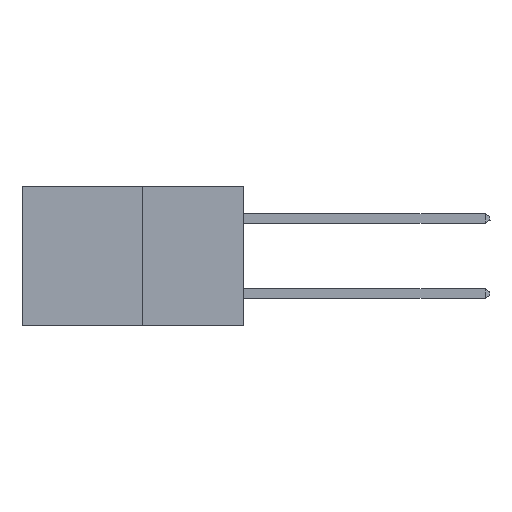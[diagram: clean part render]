
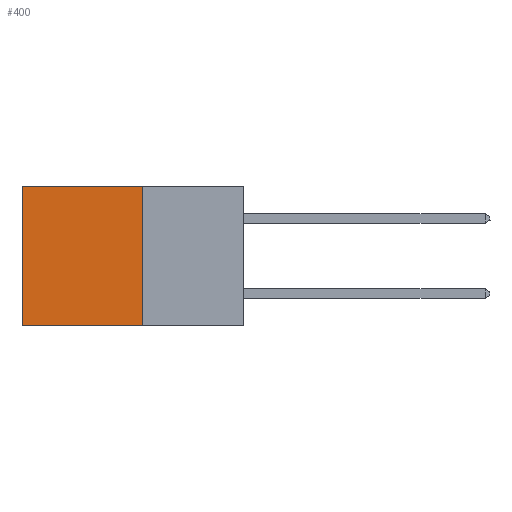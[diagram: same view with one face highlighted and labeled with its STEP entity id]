
A CAD part, left-side view. The second image highlights one B-rep face of the part: STEP entity #400.
In plain terms, the highlighted planar face has unit normal (-1, 0, 0).
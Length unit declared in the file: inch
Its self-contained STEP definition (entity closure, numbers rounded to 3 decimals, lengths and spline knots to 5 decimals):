
#313 = ORIENTED_EDGE ( 'NONE', *, *, #3958, .T. ) ;
#400 = ADVANCED_FACE ( 'NONE', ( #7407 ), #6563, .F. ) ;
#463 = EDGE_CURVE ( 'NONE', #10520, #10120, #11737, .T. ) ;
#467 = CARTESIAN_POINT ( 'NONE',  ( 0.277, 0.59, -0.37 ) ) ;
#468 = AXIS2_PLACEMENT_3D ( 'NONE', #8633, #5228, #7107 ) ;
#1292 = VECTOR ( 'NONE', #8304, 39.37008 ) ;
#1953 = VECTOR ( 'NONE', #12433, 39.37008 ) ;
#2042 = ORIENTED_EDGE ( 'NONE', *, *, #463, .F. ) ;
#2436 = EDGE_CURVE ( 'NONE', #10120, #12233, #12963, .T. ) ;
#2474 = DIRECTION ( 'NONE',  ( 0., 0., -1. ) ) ;
#2986 = DIRECTION ( 'NONE',  ( 0., 1., 0. ) ) ;
#3145 = CARTESIAN_POINT ( 'NONE',  ( 0.277, 0.27, 0. ) ) ;
#3684 = VECTOR ( 'NONE', #2986, 39.37008 ) ;
#3958 = EDGE_CURVE ( 'NONE', #10520, #4696, #11116, .T. ) ;
#4452 = ORIENTED_EDGE ( 'NONE', *, *, #11543, .T. ) ;
#4599 = CARTESIAN_POINT ( 'NONE',  ( 0.277, 0.27, -0.37 ) ) ;
#4696 = VERTEX_POINT ( 'NONE', #11150 ) ;
#5228 = DIRECTION ( 'NONE',  ( 1., 0., 0. ) ) ;
#5289 = CARTESIAN_POINT ( 'NONE',  ( 0.277, 0.27, 0. ) ) ;
#5923 = CARTESIAN_POINT ( 'NONE',  ( 0.277, 0.27, -0.37 ) ) ;
#6059 = VECTOR ( 'NONE', #2474, 39.37008 ) ;
#6563 = PLANE ( 'NONE',  #468 ) ;
#7107 = DIRECTION ( 'NONE',  ( 0., 0., -1. ) ) ;
#7407 = FACE_OUTER_BOUND ( 'NONE', #8416, .T. ) ;
#7573 = CARTESIAN_POINT ( 'NONE',  ( 0.277, 0.59, -0.37 ) ) ;
#8304 = DIRECTION ( 'NONE',  ( 0., 0., -1. ) ) ;
#8416 = EDGE_LOOP ( 'NONE', ( #4452, #12131, #2042, #313 ) ) ;
#8633 = CARTESIAN_POINT ( 'NONE',  ( 0.277, 0.27, -0.37 ) ) ;
#10120 = VERTEX_POINT ( 'NONE', #4599 ) ;
#10520 = VERTEX_POINT ( 'NONE', #3145 ) ;
#11116 = LINE ( 'NONE', #5289, #3684 ) ;
#11150 = CARTESIAN_POINT ( 'NONE',  ( 0.277, 0.59, 0. ) ) ;
#11356 = LINE ( 'NONE', #467, #6059 ) ;
#11543 = EDGE_CURVE ( 'NONE', #4696, #12233, #11356, .T. ) ;
#11737 = LINE ( 'NONE', #12634, #1292 ) ;
#12131 = ORIENTED_EDGE ( 'NONE', *, *, #2436, .F. ) ;
#12233 = VERTEX_POINT ( 'NONE', #7573 ) ;
#12433 = DIRECTION ( 'NONE',  ( 0., 1., 0. ) ) ;
#12634 = CARTESIAN_POINT ( 'NONE',  ( 0.277, 0.27, -0.37 ) ) ;
#12963 = LINE ( 'NONE', #5923, #1953 ) ;
